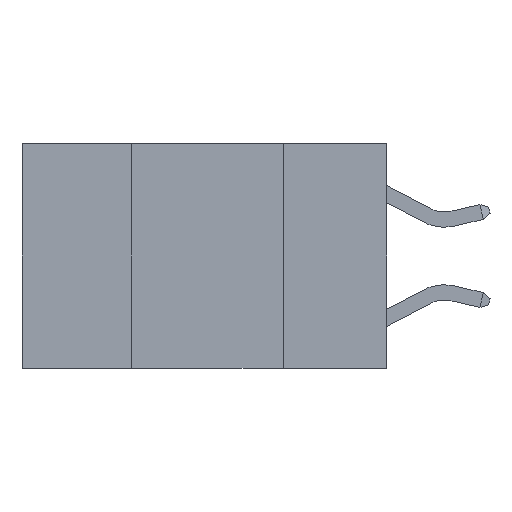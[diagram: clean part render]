
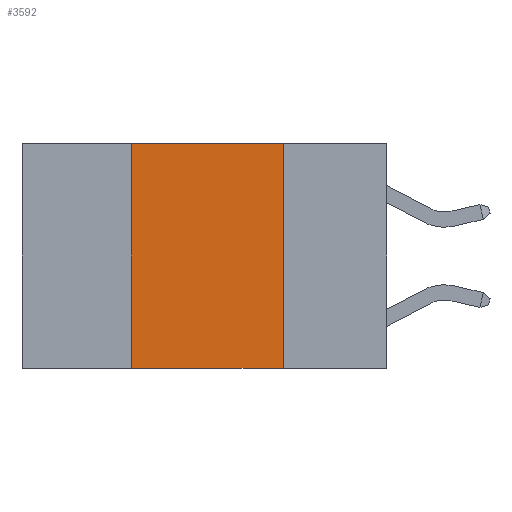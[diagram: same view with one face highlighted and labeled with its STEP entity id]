
A CAD part, left-side view. The second image highlights one B-rep face of the part: STEP entity #3592.
In plain terms, the highlighted planar face has unit normal (-1, 0, 0).
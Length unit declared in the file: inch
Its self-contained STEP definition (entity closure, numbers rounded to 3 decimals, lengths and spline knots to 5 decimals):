
#454 = LINE ( 'NONE', #6862, #1002 ) ;
#1002 = VECTOR ( 'NONE', #16660, 39.37008 ) ;
#1162 = VERTEX_POINT ( 'NONE', #13627 ) ;
#2277 = PLANE ( 'NONE',  #10320 ) ;
#2390 = DIRECTION ( 'NONE',  ( 1., 0., 0. ) ) ;
#3422 = CARTESIAN_POINT ( 'NONE',  ( 0., 0.42, 0. ) ) ;
#3592 = ADVANCED_FACE ( 'NONE', ( #15282 ), #2277, .F. ) ;
#3751 = CARTESIAN_POINT ( 'NONE',  ( 0., 0.6, 0. ) ) ;
#4931 = DIRECTION ( 'NONE',  ( 0., 0., -1. ) ) ;
#5085 = ORIENTED_EDGE ( 'NONE', *, *, #16781, .F. ) ;
#5225 = EDGE_CURVE ( 'NONE', #21048, #7466, #17746, .T. ) ;
#5454 = LINE ( 'NONE', #3751, #17103 ) ;
#6862 = CARTESIAN_POINT ( 'NONE',  ( 0., 0.42, 0. ) ) ;
#6990 = VECTOR ( 'NONE', #4931, 39.37008 ) ;
#7466 = VERTEX_POINT ( 'NONE', #8070 ) ;
#7942 = CARTESIAN_POINT ( 'NONE',  ( 0., 0.17, 0. ) ) ;
#8070 = CARTESIAN_POINT ( 'NONE',  ( 0., 0.17, -0.37 ) ) ;
#10030 = DIRECTION ( 'NONE',  ( 0., -1., 0. ) ) ;
#10176 = VECTOR ( 'NONE', #20132, 39.37008 ) ;
#10320 = AXIS2_PLACEMENT_3D ( 'NONE', #18681, #2390, #15497 ) ;
#10816 = EDGE_CURVE ( 'NONE', #1162, #7466, #17050, .T. ) ;
#13595 = EDGE_CURVE ( 'NONE', #1162, #13915, #454, .T. ) ;
#13627 = CARTESIAN_POINT ( 'NONE',  ( 0., 0.42, -0.37 ) ) ;
#13655 = CARTESIAN_POINT ( 'NONE',  ( 0., 0.6, -0.37 ) ) ;
#13691 = ORIENTED_EDGE ( 'NONE', *, *, #10816, .T. ) ;
#13915 = VERTEX_POINT ( 'NONE', #3422 ) ;
#15282 = FACE_OUTER_BOUND ( 'NONE', #16421, .T. ) ;
#15497 = DIRECTION ( 'NONE',  ( 0., 0., -1. ) ) ;
#16414 = ORIENTED_EDGE ( 'NONE', *, *, #13595, .F. ) ;
#16421 = EDGE_LOOP ( 'NONE', ( #18048, #5085, #16414, #13691 ) ) ;
#16427 = CARTESIAN_POINT ( 'NONE',  ( 0., 0.17, 0. ) ) ;
#16660 = DIRECTION ( 'NONE',  ( 0., 0., 1. ) ) ;
#16781 = EDGE_CURVE ( 'NONE', #13915, #21048, #5454, .T. ) ;
#17050 = LINE ( 'NONE', #13655, #10176 ) ;
#17103 = VECTOR ( 'NONE', #10030, 39.37008 ) ;
#17746 = LINE ( 'NONE', #7942, #6990 ) ;
#18048 = ORIENTED_EDGE ( 'NONE', *, *, #5225, .F. ) ;
#18681 = CARTESIAN_POINT ( 'NONE',  ( 0., 0.6, 0. ) ) ;
#20132 = DIRECTION ( 'NONE',  ( 0., -1., 0. ) ) ;
#21048 = VERTEX_POINT ( 'NONE', #16427 ) ;
